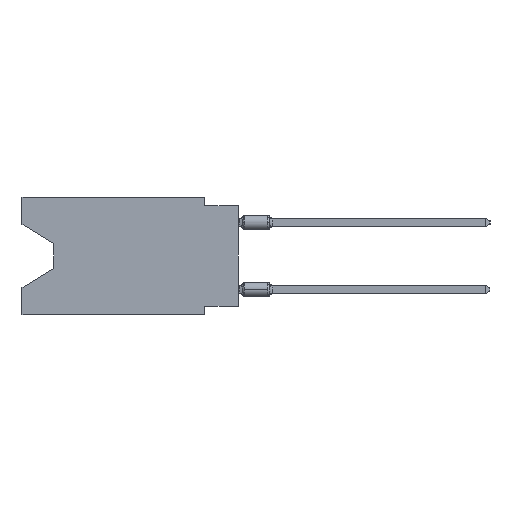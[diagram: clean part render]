
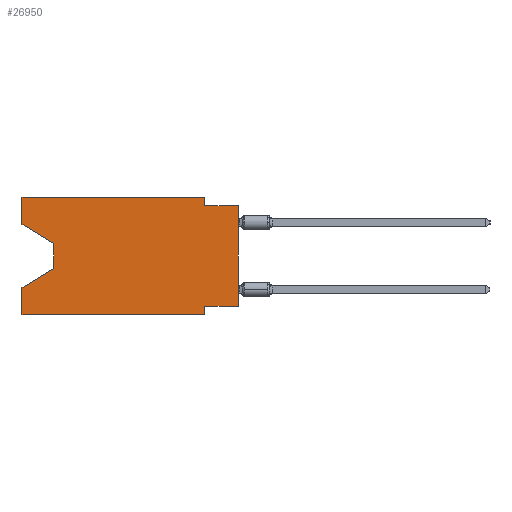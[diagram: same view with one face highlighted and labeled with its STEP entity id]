
A CAD part, left-side view. The second image highlights one B-rep face of the part: STEP entity #26950.
In plain terms, the highlighted planar face has unit normal (-1, 0, 0).
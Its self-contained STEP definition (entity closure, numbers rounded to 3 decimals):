
#1933 = DIRECTION ( 'NONE',  ( 0., 0., 1. ) ) ;
#2468 = DIRECTION ( 'NONE',  ( 0., 0., -1. ) ) ;
#2654 = CARTESIAN_POINT ( 'NONE',  ( 0., 16.383, -8.89 ) ) ;
#2952 = VERTEX_POINT ( 'NONE', #15666 ) ;
#3333 = LINE ( 'NONE', #6770, #42134 ) ;
#5085 = ORIENTED_EDGE ( 'NONE', *, *, #31128, .T. ) ;
#5616 = FACE_OUTER_BOUND ( 'NONE', #43971, .T. ) ;
#5747 = EDGE_CURVE ( 'NONE', #41168, #8946, #29479, .T. ) ;
#5828 = VECTOR ( 'NONE', #24607, 1000. ) ;
#5934 = CARTESIAN_POINT ( 'NONE',  ( 0., 16.383, 0. ) ) ;
#5959 = ORIENTED_EDGE ( 'NONE', *, *, #24986, .F. ) ;
#6140 = ORIENTED_EDGE ( 'NONE', *, *, #5747, .T. ) ;
#6770 = CARTESIAN_POINT ( 'NONE',  ( 0., 2.54, -8.89 ) ) ;
#7532 = ORIENTED_EDGE ( 'NONE', *, *, #20196, .F. ) ;
#7555 = EDGE_CURVE ( 'NONE', #23174, #47345, #9321, .T. ) ;
#7909 = VECTOR ( 'NONE', #13489, 1000. ) ;
#7977 = LINE ( 'NONE', #50802, #32447 ) ;
#8946 = VERTEX_POINT ( 'NONE', #19323 ) ;
#8962 = VECTOR ( 'NONE', #2468, 1000. ) ;
#9321 = LINE ( 'NONE', #29376, #10084 ) ;
#9792 = CARTESIAN_POINT ( 'NONE',  ( 0., 2.54, -0.635 ) ) ;
#10084 = VECTOR ( 'NONE', #1933, 1000. ) ;
#10220 = EDGE_CURVE ( 'NONE', #26243, #8946, #41432, .T. ) ;
#12010 = DIRECTION ( 'NONE',  ( 0., -0.855, -0.519 ) ) ;
#12317 = CARTESIAN_POINT ( 'NONE',  ( 0., 13.97, -5.385 ) ) ;
#13489 = DIRECTION ( 'NONE',  ( 0., 1., 0. ) ) ;
#13741 = EDGE_CURVE ( 'NONE', #39252, #32687, #7977, .T. ) ;
#13827 = PLANE ( 'NONE',  #28178 ) ;
#15429 = CARTESIAN_POINT ( 'NONE',  ( 0., 13.97, -3.505 ) ) ;
#15666 = CARTESIAN_POINT ( 'NONE',  ( 0., 2.54, -8.255 ) ) ;
#15972 = LINE ( 'NONE', #48145, #47413 ) ;
#17229 = DIRECTION ( 'NONE',  ( 0., 0.855, -0.519 ) ) ;
#17779 = CARTESIAN_POINT ( 'NONE',  ( 0., 16.383, 0. ) ) ;
#17888 = EDGE_CURVE ( 'NONE', #2952, #32687, #3333, .T. ) ;
#18004 = VERTEX_POINT ( 'NONE', #12317 ) ;
#18009 = LINE ( 'NONE', #41193, #39446 ) ;
#19133 = ORIENTED_EDGE ( 'NONE', *, *, #33925, .F. ) ;
#19323 = CARTESIAN_POINT ( 'NONE',  ( 0., 0., -0.635 ) ) ;
#20196 = EDGE_CURVE ( 'NONE', #24146, #26243, #28463, .T. ) ;
#20353 = VECTOR ( 'NONE', #38355, 1000. ) ;
#21315 = CARTESIAN_POINT ( 'NONE',  ( 0., 0., -8.255 ) ) ;
#21821 = DIRECTION ( 'NONE',  ( 0., 0., 1. ) ) ;
#22088 = CARTESIAN_POINT ( 'NONE',  ( 0., 0., 0. ) ) ;
#22261 = DIRECTION ( 'NONE',  ( 0., 0., -1. ) ) ;
#22796 = LINE ( 'NONE', #38587, #8962 ) ;
#22898 = DIRECTION ( 'NONE',  ( 0., 0., -1. ) ) ;
#23174 = VERTEX_POINT ( 'NONE', #38128 ) ;
#24146 = VERTEX_POINT ( 'NONE', #50262 ) ;
#24149 = ORIENTED_EDGE ( 'NONE', *, *, #7555, .F. ) ;
#24607 = DIRECTION ( 'NONE',  ( 0., -1., 0. ) ) ;
#24986 = EDGE_CURVE ( 'NONE', #41168, #2952, #41919, .T. ) ;
#25459 = VERTEX_POINT ( 'NONE', #15429 ) ;
#26243 = VERTEX_POINT ( 'NONE', #9792 ) ;
#26267 = VERTEX_POINT ( 'NONE', #33259 ) ;
#26471 = DIRECTION ( 'NONE',  ( 1., 0., 0. ) ) ;
#26950 = ADVANCED_FACE ( 'NONE', ( #5616 ), #13827, .F. ) ;
#28178 = AXIS2_PLACEMENT_3D ( 'NONE', #17779, #26471, #22261 ) ;
#28293 = DIRECTION ( 'NONE',  ( 0., -1., 0. ) ) ;
#28463 = LINE ( 'NONE', #40561, #32267 ) ;
#29101 = LINE ( 'NONE', #33050, #43016 ) ;
#29376 = CARTESIAN_POINT ( 'NONE',  ( 0., 16.383, 0. ) ) ;
#29479 = LINE ( 'NONE', #22088, #48637 ) ;
#29501 = ORIENTED_EDGE ( 'NONE', *, *, #41814, .T. ) ;
#31128 = EDGE_CURVE ( 'NONE', #18004, #26267, #18009, .T. ) ;
#32267 = VECTOR ( 'NONE', #32669, 1000. ) ;
#32447 = VECTOR ( 'NONE', #28293, 1000. ) ;
#32669 = DIRECTION ( 'NONE',  ( 0., 0., -1. ) ) ;
#32687 = VERTEX_POINT ( 'NONE', #45807 ) ;
#33050 = CARTESIAN_POINT ( 'NONE',  ( 0., 16.383, 0. ) ) ;
#33259 = CARTESIAN_POINT ( 'NONE',  ( 0., 16.383, -6.852 ) ) ;
#33400 = ORIENTED_EDGE ( 'NONE', *, *, #13741, .T. ) ;
#33556 = DIRECTION ( 'NONE',  ( 0., 0., 1. ) ) ;
#33925 = EDGE_CURVE ( 'NONE', #39252, #26267, #29101, .T. ) ;
#34698 = EDGE_CURVE ( 'NONE', #47345, #24146, #41266, .T. ) ;
#37111 = ORIENTED_EDGE ( 'NONE', *, *, #10220, .F. ) ;
#37453 = EDGE_CURVE ( 'NONE', #23174, #25459, #15972, .T. ) ;
#38128 = CARTESIAN_POINT ( 'NONE',  ( 0., 16.383, -2.038 ) ) ;
#38355 = DIRECTION ( 'NONE',  ( 0., -1., 0. ) ) ;
#38587 = CARTESIAN_POINT ( 'NONE',  ( 0., 13.97, -3.505 ) ) ;
#38914 = ORIENTED_EDGE ( 'NONE', *, *, #34698, .F. ) ;
#39252 = VERTEX_POINT ( 'NONE', #2654 ) ;
#39446 = VECTOR ( 'NONE', #17229, 1000. ) ;
#39753 = ORIENTED_EDGE ( 'NONE', *, *, #17888, .F. ) ;
#40561 = CARTESIAN_POINT ( 'NONE',  ( 0., 2.54, 0. ) ) ;
#40647 = CARTESIAN_POINT ( 'NONE',  ( 0., 0., -0.635 ) ) ;
#41168 = VERTEX_POINT ( 'NONE', #21315 ) ;
#41193 = CARTESIAN_POINT ( 'NONE',  ( 0., 13.97, -5.385 ) ) ;
#41266 = LINE ( 'NONE', #5934, #20353 ) ;
#41432 = LINE ( 'NONE', #40647, #5828 ) ;
#41814 = EDGE_CURVE ( 'NONE', #25459, #18004, #22796, .T. ) ;
#41919 = LINE ( 'NONE', #42183, #7909 ) ;
#42134 = VECTOR ( 'NONE', #22898, 1000. ) ;
#42183 = CARTESIAN_POINT ( 'NONE',  ( 0., 0., -8.255 ) ) ;
#43016 = VECTOR ( 'NONE', #33556, 1000. ) ;
#43971 = EDGE_LOOP ( 'NONE', ( #48917, #29501, #5085, #19133, #33400, #39753, #5959, #6140, #37111, #7532, #38914, #24149 ) ) ;
#45807 = CARTESIAN_POINT ( 'NONE',  ( 0., 2.54, -8.89 ) ) ;
#47345 = VERTEX_POINT ( 'NONE', #50629 ) ;
#47413 = VECTOR ( 'NONE', #12010, 1000. ) ;
#48145 = CARTESIAN_POINT ( 'NONE',  ( 0., 16.383, -2.038 ) ) ;
#48637 = VECTOR ( 'NONE', #21821, 1000. ) ;
#48917 = ORIENTED_EDGE ( 'NONE', *, *, #37453, .T. ) ;
#50262 = CARTESIAN_POINT ( 'NONE',  ( 0., 2.54, 0. ) ) ;
#50629 = CARTESIAN_POINT ( 'NONE',  ( 0., 16.383, 0. ) ) ;
#50802 = CARTESIAN_POINT ( 'NONE',  ( 0., 16.383, -8.89 ) ) ;
